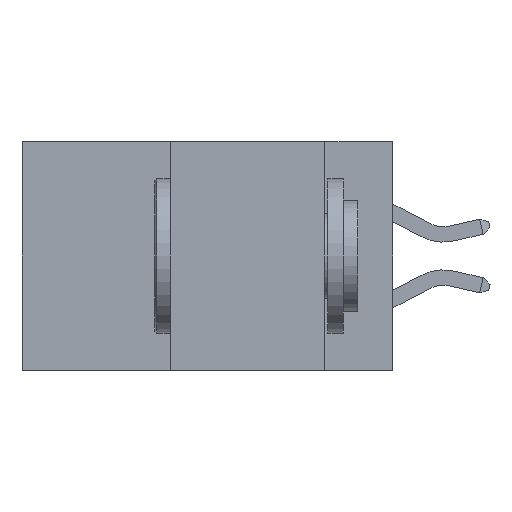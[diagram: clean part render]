
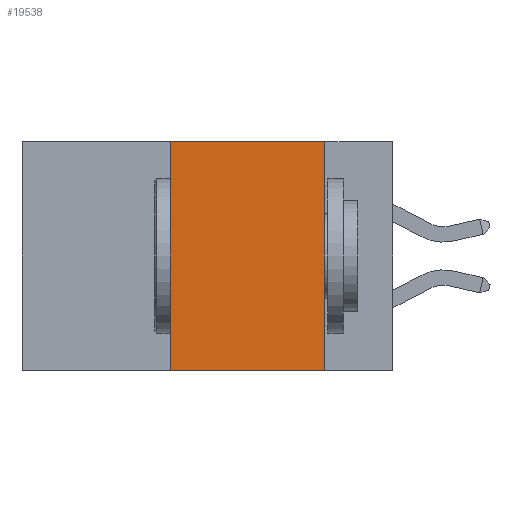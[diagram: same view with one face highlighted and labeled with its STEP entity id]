
A CAD part, left-side view. The second image highlights one B-rep face of the part: STEP entity #19538.
In plain terms, the highlighted planar face has unit normal (-1, 0, 0).
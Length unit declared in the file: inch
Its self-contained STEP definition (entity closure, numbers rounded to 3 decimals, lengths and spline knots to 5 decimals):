
#813 = EDGE_CURVE ( 'NONE', #5336, #12423, #9506, .T. ) ;
#1011 = EDGE_LOOP ( 'NONE', ( #25605, #21518, #22134, #11834 ) ) ;
#2090 = CARTESIAN_POINT ( 'NONE',  ( 0., 0.11, 0. ) ) ;
#3529 = VERTEX_POINT ( 'NONE', #2090 ) ;
#4315 = EDGE_CURVE ( 'NONE', #3529, #4686, #21449, .T. ) ;
#4679 = VECTOR ( 'NONE', #8769, 39.37008 ) ;
#4686 = VERTEX_POINT ( 'NONE', #4691 ) ;
#4691 = CARTESIAN_POINT ( 'NONE',  ( 0., 0.11, -0.37 ) ) ;
#5106 = PLANE ( 'NONE',  #12711 ) ;
#5336 = VERTEX_POINT ( 'NONE', #13759 ) ;
#5648 = CARTESIAN_POINT ( 'NONE',  ( 0., 0.11, 0. ) ) ;
#5855 = DIRECTION ( 'NONE',  ( 0., 0., -1. ) ) ;
#6997 = VECTOR ( 'NONE', #11479, 39.37008 ) ;
#7199 = DIRECTION ( 'NONE',  ( 0., 0., -1. ) ) ;
#7661 = LINE ( 'NONE', #9331, #6997 ) ;
#8769 = DIRECTION ( 'NONE',  ( 0., -1., 0. ) ) ;
#9331 = CARTESIAN_POINT ( 'NONE',  ( 0., 0.6, 0. ) ) ;
#9506 = LINE ( 'NONE', #23678, #15797 ) ;
#10289 = LINE ( 'NONE', #23228, #4679 ) ;
#11479 = DIRECTION ( 'NONE',  ( 0., -1., 0. ) ) ;
#11834 = ORIENTED_EDGE ( 'NONE', *, *, #26359, .T. ) ;
#12423 = VERTEX_POINT ( 'NONE', #21312 ) ;
#12711 = AXIS2_PLACEMENT_3D ( 'NONE', #13499, #19754, #7199 ) ;
#13499 = CARTESIAN_POINT ( 'NONE',  ( 0., 0.6, 0. ) ) ;
#13759 = CARTESIAN_POINT ( 'NONE',  ( 0., 0.36, -0.37 ) ) ;
#15097 = EDGE_CURVE ( 'NONE', #12423, #3529, #7661, .T. ) ;
#15797 = VECTOR ( 'NONE', #23178, 39.37008 ) ;
#16045 = VECTOR ( 'NONE', #5855, 39.37008 ) ;
#19538 = ADVANCED_FACE ( 'NONE', ( #23414 ), #5106, .F. ) ;
#19754 = DIRECTION ( 'NONE',  ( 1., 0., 0. ) ) ;
#21312 = CARTESIAN_POINT ( 'NONE',  ( 0., 0.36, 0. ) ) ;
#21449 = LINE ( 'NONE', #5648, #16045 ) ;
#21518 = ORIENTED_EDGE ( 'NONE', *, *, #15097, .F. ) ;
#22134 = ORIENTED_EDGE ( 'NONE', *, *, #813, .F. ) ;
#23178 = DIRECTION ( 'NONE',  ( 0., 0., 1. ) ) ;
#23228 = CARTESIAN_POINT ( 'NONE',  ( 0., 0.6, -0.37 ) ) ;
#23414 = FACE_OUTER_BOUND ( 'NONE', #1011, .T. ) ;
#23678 = CARTESIAN_POINT ( 'NONE',  ( 0., 0.36, 0. ) ) ;
#25605 = ORIENTED_EDGE ( 'NONE', *, *, #4315, .F. ) ;
#26359 = EDGE_CURVE ( 'NONE', #5336, #4686, #10289, .T. ) ;
